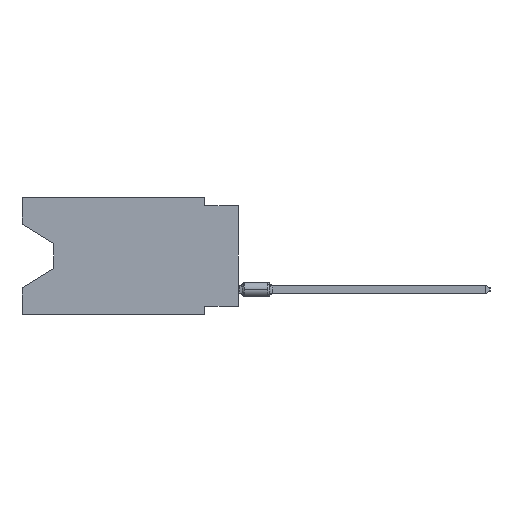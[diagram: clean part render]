
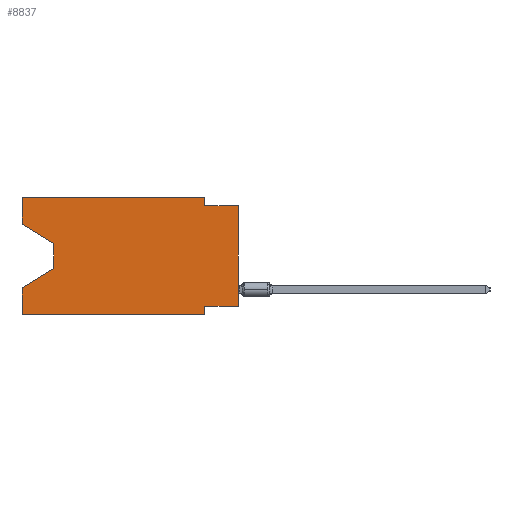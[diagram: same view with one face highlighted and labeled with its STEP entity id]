
A CAD part, left-side view. The second image highlights one B-rep face of the part: STEP entity #8837.
In plain terms, the highlighted planar face has unit normal (-1, 0, 0).
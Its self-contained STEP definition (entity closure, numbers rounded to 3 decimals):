
#441 = DIRECTION ( 'NONE',  ( 0., 0., 1. ) ) ;
#536 = DIRECTION ( 'NONE',  ( 0., 0.855, -0.519 ) ) ;
#805 = LINE ( 'NONE', #16068, #7252 ) ;
#1277 = CARTESIAN_POINT ( 'NONE',  ( 0., 0., -8.255 ) ) ;
#2073 = CARTESIAN_POINT ( 'NONE',  ( 0., 16.383, -8.89 ) ) ;
#3607 = ORIENTED_EDGE ( 'NONE', *, *, #6700, .F. ) ;
#4011 = DIRECTION ( 'NONE',  ( 0., 0., -1. ) ) ;
#4020 = CARTESIAN_POINT ( 'NONE',  ( 0., 16.383, 0. ) ) ;
#4120 = VECTOR ( 'NONE', #35372, 1000. ) ;
#4293 = CARTESIAN_POINT ( 'NONE',  ( 0., 16.383, 0. ) ) ;
#4733 = ORIENTED_EDGE ( 'NONE', *, *, #8397, .F. ) ;
#4742 = ORIENTED_EDGE ( 'NONE', *, *, #12422, .T. ) ;
#5505 = EDGE_CURVE ( 'NONE', #19342, #29581, #20077, .T. ) ;
#5628 = LINE ( 'NONE', #25030, #34927 ) ;
#5974 = VECTOR ( 'NONE', #28947, 1000. ) ;
#6610 = FACE_OUTER_BOUND ( 'NONE', #19752, .T. ) ;
#6700 = EDGE_CURVE ( 'NONE', #34629, #20447, #35347, .T. ) ;
#6798 = LINE ( 'NONE', #32292, #14866 ) ;
#7019 = PLANE ( 'NONE',  #41314 ) ;
#7252 = VECTOR ( 'NONE', #26485, 1000. ) ;
#8070 = CARTESIAN_POINT ( 'NONE',  ( 0., 2.54, -0.635 ) ) ;
#8128 = ORIENTED_EDGE ( 'NONE', *, *, #31553, .F. ) ;
#8397 = EDGE_CURVE ( 'NONE', #25487, #40404, #805, .T. ) ;
#8506 = CARTESIAN_POINT ( 'NONE',  ( 0., 13.97, -3.505 ) ) ;
#8575 = VERTEX_POINT ( 'NONE', #11234 ) ;
#8594 = CARTESIAN_POINT ( 'NONE',  ( 0., 2.54, -8.89 ) ) ;
#8650 = CARTESIAN_POINT ( 'NONE',  ( 0., 16.383, -8.89 ) ) ;
#8837 = ADVANCED_FACE ( 'NONE', ( #6610 ), #7019, .F. ) ;
#9168 = DIRECTION ( 'NONE',  ( 0., 0., 1. ) ) ;
#9330 = ORIENTED_EDGE ( 'NONE', *, *, #26856, .T. ) ;
#10702 = CARTESIAN_POINT ( 'NONE',  ( 0., 16.383, -2.038 ) ) ;
#11234 = CARTESIAN_POINT ( 'NONE',  ( 0., 0., -0.635 ) ) ;
#11236 = VECTOR ( 'NONE', #37270, 1000. ) ;
#11456 = EDGE_CURVE ( 'NONE', #29581, #15098, #16138, .T. ) ;
#11721 = EDGE_CURVE ( 'NONE', #41249, #20838, #13216, .T. ) ;
#11983 = CARTESIAN_POINT ( 'NONE',  ( 0., 2.54, -8.255 ) ) ;
#12244 = ORIENTED_EDGE ( 'NONE', *, *, #40857, .T. ) ;
#12422 = EDGE_CURVE ( 'NONE', #26041, #20838, #6798, .T. ) ;
#13216 = LINE ( 'NONE', #4020, #4120 ) ;
#13631 = CARTESIAN_POINT ( 'NONE',  ( 0., 2.54, 0. ) ) ;
#14802 = EDGE_CURVE ( 'NONE', #40404, #8575, #14829, .T. ) ;
#14829 = LINE ( 'NONE', #23389, #16939 ) ;
#14866 = VECTOR ( 'NONE', #536, 1000. ) ;
#15098 = VERTEX_POINT ( 'NONE', #8594 ) ;
#15394 = LINE ( 'NONE', #8506, #30789 ) ;
#16068 = CARTESIAN_POINT ( 'NONE',  ( 0., 2.54, 0. ) ) ;
#16138 = LINE ( 'NONE', #28871, #32817 ) ;
#16638 = DIRECTION ( 'NONE',  ( 1., 0., 0. ) ) ;
#16939 = VECTOR ( 'NONE', #36132, 1000. ) ;
#17825 = VERTEX_POINT ( 'NONE', #38694 ) ;
#19342 = VERTEX_POINT ( 'NONE', #38059 ) ;
#19354 = DIRECTION ( 'NONE',  ( 0., 0., -1. ) ) ;
#19752 = EDGE_LOOP ( 'NONE', ( #20916, #20135, #4742, #33677, #12244, #24583, #30906, #9330, #29028, #4733, #8128, #3607 ) ) ;
#19755 = CARTESIAN_POINT ( 'NONE',  ( 0., 16.383, 0. ) ) ;
#19860 = CARTESIAN_POINT ( 'NONE',  ( 0., 16.383, 0. ) ) ;
#20077 = LINE ( 'NONE', #1277, #34444 ) ;
#20135 = ORIENTED_EDGE ( 'NONE', *, *, #21177, .T. ) ;
#20447 = VERTEX_POINT ( 'NONE', #4293 ) ;
#20822 = CARTESIAN_POINT ( 'NONE',  ( 0., 16.383, -6.852 ) ) ;
#20838 = VERTEX_POINT ( 'NONE', #20822 ) ;
#20916 = ORIENTED_EDGE ( 'NONE', *, *, #23411, .T. ) ;
#21177 = EDGE_CURVE ( 'NONE', #17825, #26041, #15394, .T. ) ;
#22431 = VECTOR ( 'NONE', #441, 1000. ) ;
#23389 = CARTESIAN_POINT ( 'NONE',  ( 0., 0., -0.635 ) ) ;
#23411 = EDGE_CURVE ( 'NONE', #34629, #17825, #5628, .T. ) ;
#23617 = DIRECTION ( 'NONE',  ( 0., 1., 0. ) ) ;
#24583 = ORIENTED_EDGE ( 'NONE', *, *, #11456, .F. ) ;
#24830 = DIRECTION ( 'NONE',  ( 0., -0.855, -0.519 ) ) ;
#25030 = CARTESIAN_POINT ( 'NONE',  ( 0., 16.383, -2.038 ) ) ;
#25176 = CARTESIAN_POINT ( 'NONE',  ( 0., 13.97, -5.385 ) ) ;
#25487 = VERTEX_POINT ( 'NONE', #13631 ) ;
#26041 = VERTEX_POINT ( 'NONE', #25176 ) ;
#26085 = VECTOR ( 'NONE', #9168, 1000. ) ;
#26485 = DIRECTION ( 'NONE',  ( 0., 0., -1. ) ) ;
#26856 = EDGE_CURVE ( 'NONE', #19342, #8575, #37396, .T. ) ;
#28871 = CARTESIAN_POINT ( 'NONE',  ( 0., 2.54, -8.89 ) ) ;
#28947 = DIRECTION ( 'NONE',  ( 0., -1., 0. ) ) ;
#29028 = ORIENTED_EDGE ( 'NONE', *, *, #14802, .F. ) ;
#29365 = CARTESIAN_POINT ( 'NONE',  ( 0., 16.383, 0. ) ) ;
#29581 = VERTEX_POINT ( 'NONE', #11983 ) ;
#30789 = VECTOR ( 'NONE', #40693, 1000. ) ;
#30906 = ORIENTED_EDGE ( 'NONE', *, *, #5505, .F. ) ;
#31122 = CARTESIAN_POINT ( 'NONE',  ( 0., 0., 0. ) ) ;
#31553 = EDGE_CURVE ( 'NONE', #20447, #25487, #35844, .T. ) ;
#32292 = CARTESIAN_POINT ( 'NONE',  ( 0., 13.97, -5.385 ) ) ;
#32817 = VECTOR ( 'NONE', #4011, 1000. ) ;
#33677 = ORIENTED_EDGE ( 'NONE', *, *, #11721, .F. ) ;
#34444 = VECTOR ( 'NONE', #23617, 1000. ) ;
#34629 = VERTEX_POINT ( 'NONE', #10702 ) ;
#34927 = VECTOR ( 'NONE', #24830, 1000. ) ;
#35347 = LINE ( 'NONE', #19860, #22431 ) ;
#35372 = DIRECTION ( 'NONE',  ( 0., 0., 1. ) ) ;
#35844 = LINE ( 'NONE', #29365, #5974 ) ;
#36132 = DIRECTION ( 'NONE',  ( 0., -1., 0. ) ) ;
#37270 = DIRECTION ( 'NONE',  ( 0., -1., 0. ) ) ;
#37396 = LINE ( 'NONE', #31122, #26085 ) ;
#38059 = CARTESIAN_POINT ( 'NONE',  ( 0., 0., -8.255 ) ) ;
#38694 = CARTESIAN_POINT ( 'NONE',  ( 0., 13.97, -3.505 ) ) ;
#40404 = VERTEX_POINT ( 'NONE', #8070 ) ;
#40621 = LINE ( 'NONE', #8650, #11236 ) ;
#40693 = DIRECTION ( 'NONE',  ( 0., 0., -1. ) ) ;
#40857 = EDGE_CURVE ( 'NONE', #41249, #15098, #40621, .T. ) ;
#41249 = VERTEX_POINT ( 'NONE', #2073 ) ;
#41314 = AXIS2_PLACEMENT_3D ( 'NONE', #19755, #16638, #19354 ) ;
